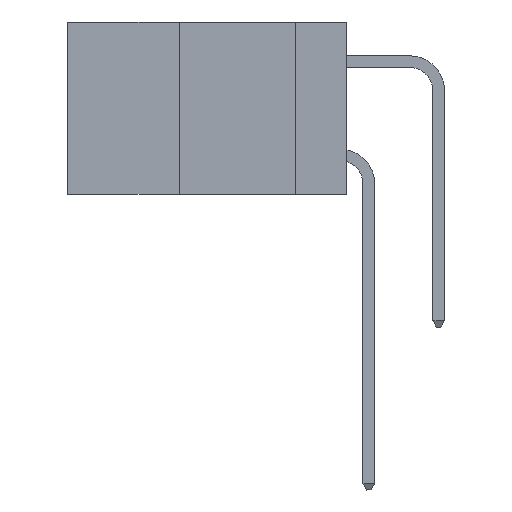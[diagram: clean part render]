
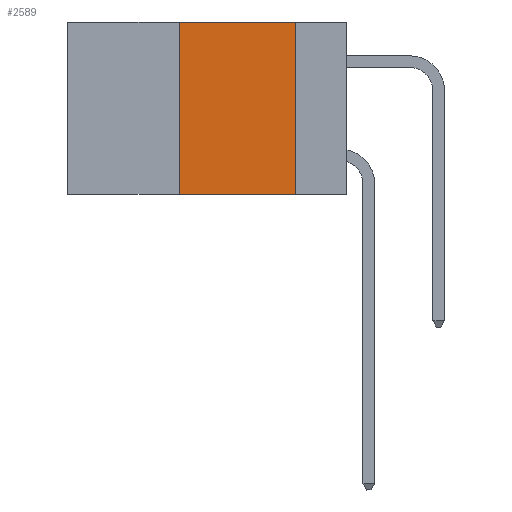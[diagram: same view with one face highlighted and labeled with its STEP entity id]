
A CAD part, left-side view. The second image highlights one B-rep face of the part: STEP entity #2589.
In plain terms, the highlighted planar face has unit normal (-1, 0, 0).
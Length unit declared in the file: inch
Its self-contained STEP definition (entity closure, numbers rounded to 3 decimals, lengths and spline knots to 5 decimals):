
#125 = CARTESIAN_POINT ( 'NONE',  ( 0., 0.6, 0. ) ) ;
#365 = DIRECTION ( 'NONE',  ( 0., 0., -1. ) ) ;
#684 = CARTESIAN_POINT ( 'NONE',  ( 0., 0.11, 0. ) ) ;
#991 = CARTESIAN_POINT ( 'NONE',  ( 0., 0.36, -0.37 ) ) ;
#1382 = EDGE_LOOP ( 'NONE', ( #10487, #12540, #2358, #7876 ) ) ;
#1384 = DIRECTION ( 'NONE',  ( 0., -1., 0. ) ) ;
#2074 = CARTESIAN_POINT ( 'NONE',  ( 0., 0.36, 0. ) ) ;
#2358 = ORIENTED_EDGE ( 'NONE', *, *, #7432, .F. ) ;
#2383 = FACE_OUTER_BOUND ( 'NONE', #1382, .T. ) ;
#2589 = ADVANCED_FACE ( 'NONE', ( #2383 ), #10400, .F. ) ;
#3323 = DIRECTION ( 'NONE',  ( 0., 0., 1. ) ) ;
#5001 = VERTEX_POINT ( 'NONE', #684 ) ;
#5848 = CARTESIAN_POINT ( 'NONE',  ( 0., 0.6, -0.37 ) ) ;
#6191 = EDGE_CURVE ( 'NONE', #13488, #12236, #11850, .T. ) ;
#6212 = AXIS2_PLACEMENT_3D ( 'NONE', #8859, #8910, #8491 ) ;
#7080 = VERTEX_POINT ( 'NONE', #7551 ) ;
#7086 = DIRECTION ( 'NONE',  ( 0., -1., 0. ) ) ;
#7432 = EDGE_CURVE ( 'NONE', #13488, #7080, #14781, .T. ) ;
#7551 = CARTESIAN_POINT ( 'NONE',  ( 0., 0.36, 0. ) ) ;
#7876 = ORIENTED_EDGE ( 'NONE', *, *, #6191, .T. ) ;
#8110 = LINE ( 'NONE', #125, #14195 ) ;
#8256 = CARTESIAN_POINT ( 'NONE',  ( 0., 0.11, -0.37 ) ) ;
#8369 = VECTOR ( 'NONE', #3323, 39.37008 ) ;
#8491 = DIRECTION ( 'NONE',  ( 0., 0., -1. ) ) ;
#8859 = CARTESIAN_POINT ( 'NONE',  ( 0., 0.6, 0. ) ) ;
#8910 = DIRECTION ( 'NONE',  ( 1., 0., 0. ) ) ;
#9758 = EDGE_CURVE ( 'NONE', #7080, #5001, #8110, .T. ) ;
#10400 = PLANE ( 'NONE',  #6212 ) ;
#10487 = ORIENTED_EDGE ( 'NONE', *, *, #11104, .F. ) ;
#11104 = EDGE_CURVE ( 'NONE', #5001, #12236, #14148, .T. ) ;
#11850 = LINE ( 'NONE', #5848, #14664 ) ;
#12236 = VERTEX_POINT ( 'NONE', #8256 ) ;
#12540 = ORIENTED_EDGE ( 'NONE', *, *, #9758, .F. ) ;
#12573 = CARTESIAN_POINT ( 'NONE',  ( 0., 0.11, 0. ) ) ;
#13488 = VERTEX_POINT ( 'NONE', #991 ) ;
#13756 = VECTOR ( 'NONE', #365, 39.37008 ) ;
#14148 = LINE ( 'NONE', #12573, #13756 ) ;
#14195 = VECTOR ( 'NONE', #1384, 39.37008 ) ;
#14664 = VECTOR ( 'NONE', #7086, 39.37008 ) ;
#14781 = LINE ( 'NONE', #2074, #8369 ) ;
